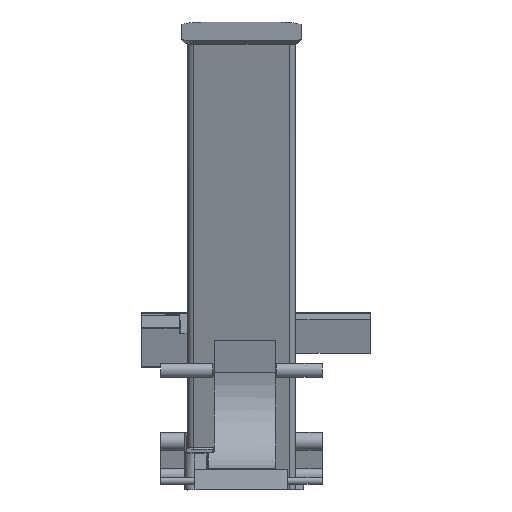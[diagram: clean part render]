
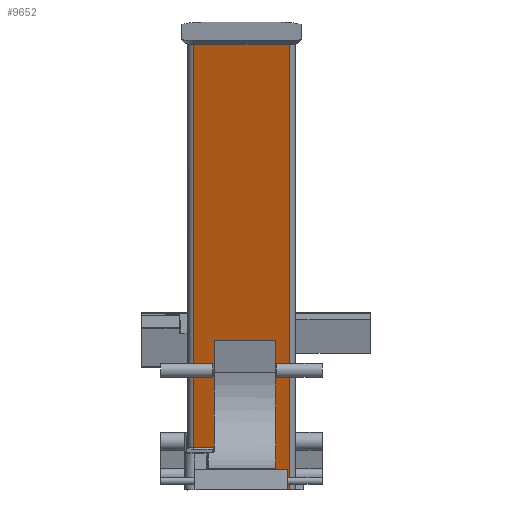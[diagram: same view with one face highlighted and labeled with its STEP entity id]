
A CAD part, left-side view. The second image highlights one B-rep face of the part: STEP entity #9652.
In plain terms, the highlighted planar face has unit normal (-0.951, 0, -0.309).
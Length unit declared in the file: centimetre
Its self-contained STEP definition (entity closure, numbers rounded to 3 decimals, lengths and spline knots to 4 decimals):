
#1104=ELLIPSE($,#10284,0.0279,0.0265);
#1105=ELLIPSE($,#10285,0.0279,0.0265);
#1236=FACE_OUTER_BOUND($,#1868,.T.);
#1868=EDGE_LOOP($,(#6496,#6497,#6498,#6499,#6500,#6501,#6502,#6503,#6504));
#2713=LINE($,#14660,#3347);
#2731=LINE($,#14890,#3365);
#2732=LINE($,#14892,#3366);
#2733=LINE($,#14894,#3367);
#2734=LINE($,#14898,#3368);
#2735=LINE($,#14902,#3369);
#2736=LINE($,#14903,#3370);
#3347=VECTOR($,#11496,2.142);
#3365=VECTOR($,#11528,9.4725);
#3366=VECTOR($,#11529,0.5861);
#3367=VECTOR($,#11530,0.3878);
#3368=VECTOR($,#11533,0.7784);
#3369=VECTOR($,#11536,0.9926);
#3370=VECTOR($,#11537,10.4518);
#3991=VERTEX_POINT($,#14657);
#3992=VERTEX_POINT($,#14659);
#4007=VERTEX_POINT($,#14889);
#4008=VERTEX_POINT($,#14891);
#4009=VERTEX_POINT($,#14893);
#4010=VERTEX_POINT($,#14895);
#4011=VERTEX_POINT($,#14897);
#4012=VERTEX_POINT($,#14899);
#4013=VERTEX_POINT($,#14901);
#4917=EDGE_CURVE($,#3992,#3991,#2713,.T.);
#4945=EDGE_CURVE($,#3991,#4007,#2731,.T.);
#4946=EDGE_CURVE($,#4007,#4008,#2732,.T.);
#4947=EDGE_CURVE($,#4009,#4008,#2733,.T.);
#4948=EDGE_CURVE($,#4009,#4010,#1104,.T.);
#4949=EDGE_CURVE($,#4010,#4011,#2734,.T.);
#4950=EDGE_CURVE($,#4011,#4012,#1105,.T.);
#4951=EDGE_CURVE($,#4012,#4013,#2735,.T.);
#4952=EDGE_CURVE($,#3992,#4013,#2736,.T.);
#6496=ORIENTED_EDGE($,*,*,#4917,.T.);
#6497=ORIENTED_EDGE($,*,*,#4945,.T.);
#6498=ORIENTED_EDGE($,*,*,#4946,.T.);
#6499=ORIENTED_EDGE($,*,*,#4947,.F.);
#6500=ORIENTED_EDGE($,*,*,#4948,.T.);
#6501=ORIENTED_EDGE($,*,*,#4949,.T.);
#6502=ORIENTED_EDGE($,*,*,#4950,.T.);
#6503=ORIENTED_EDGE($,*,*,#4951,.T.);
#6504=ORIENTED_EDGE($,*,*,#4952,.F.);
#9487=PLANE($,#10283);
#9652=ADVANCED_FACE($,(#1236),#9487,.T.);
#10283=AXIS2_PLACEMENT_3D($,#14888,#11526,#11527);
#10284=AXIS2_PLACEMENT_3D($,#14896,#11531,#11532);
#10285=AXIS2_PLACEMENT_3D($,#14900,#11534,#11535);
#11496=DIRECTION($,(0.,1.,0.));
#11526=DIRECTION('center_axis',(-0.951,0.,-0.309));
#11527=DIRECTION('ref_axis',(0.,1.,0.));
#11528=DIRECTION($,(0.309,0.,-0.951));
#11529=DIRECTION($,(0.,-1.,0.));
#11530=DIRECTION($,(-0.309,0.,0.951));
#11531=DIRECTION('center_axis',(-0.951,0.,-0.309));
#11532=DIRECTION('ref_axis',(0.309,0.,-0.951));
#11533=DIRECTION($,(0.224,-0.69,-0.689));
#11534=DIRECTION('center_axis',(-0.951,0.,-0.309));
#11535=DIRECTION('ref_axis',(0.309,0.,-0.951));
#11536=DIRECTION($,(0.,-1.,0.));
#11537=DIRECTION($,(0.309,0.,-0.951));
#14657=CARTESIAN_POINT('',(-7.7988,11.046,5.9458));
#14659=CARTESIAN_POINT('',(-7.7988,8.904,5.9458));
#14660=CARTESIAN_POINT($,(-7.7988,9.3758,5.9458));
#14888=CARTESIAN_POINT('Origin',(-7.5733,8.7765,5.2517));
#14889=CARTESIAN_POINT('',(-4.8717,11.046,-3.0631));
#14890=CARTESIAN_POINT($,(-7.5733,11.046,5.2517));
#14891=CARTESIAN_POINT('',(-4.8717,10.4599,-3.0631));
#14892=CARTESIAN_POINT($,(-4.8717,9.7583,-3.0631));
#14893=CARTESIAN_POINT('',(-4.7518,10.4599,-3.4319));
#14894=CARTESIAN_POINT($,(-6.1579,10.4599,0.8956));
#14895=CARTESIAN_POINT('',(-4.7457,10.4521,-3.4506));
#14896=CARTESIAN_POINT('Origin',(-4.7518,10.4334,-3.4319));
#14897=CARTESIAN_POINT('',(-4.5716,9.9153,-3.9867));
#14898=CARTESIAN_POINT($,(-5.2673,12.0593,-1.8456));
#14899=CARTESIAN_POINT('',(-4.569,9.8966,-3.9944));
#14900=CARTESIAN_POINT('Origin',(-4.5777,9.8966,-3.9679));
#14901=CARTESIAN_POINT('',(-4.569,8.904,-3.9944));
#14902=CARTESIAN_POINT($,(-4.569,9.3758,-3.9944));
#14903=CARTESIAN_POINT($,(-7.5733,8.904,5.2517));
